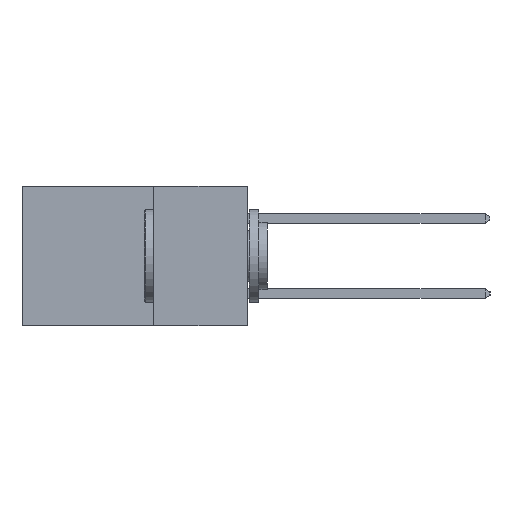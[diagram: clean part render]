
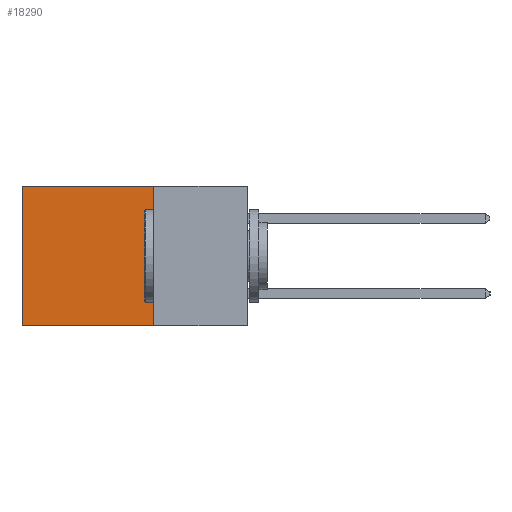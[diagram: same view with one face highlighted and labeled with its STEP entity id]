
A CAD part, left-side view. The second image highlights one B-rep face of the part: STEP entity #18290.
In plain terms, the highlighted planar face has unit normal (-1, 0, 0).
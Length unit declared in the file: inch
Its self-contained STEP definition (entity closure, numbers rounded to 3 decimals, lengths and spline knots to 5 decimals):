
#93 = DIRECTION ( 'NONE',  ( 0., 1., 0. ) ) ;
#675 = CARTESIAN_POINT ( 'NONE',  ( 0.2615, 0.25, -0.37 ) ) ;
#1195 = LINE ( 'NONE', #4726, #13088 ) ;
#2141 = LINE ( 'NONE', #5996, #18094 ) ;
#2378 = VERTEX_POINT ( 'NONE', #8078 ) ;
#2873 = CARTESIAN_POINT ( 'NONE',  ( 0.2615, 0.25, -0.37 ) ) ;
#2901 = DIRECTION ( 'NONE',  ( 0., 0., -1. ) ) ;
#3319 = AXIS2_PLACEMENT_3D ( 'NONE', #675, #13069, #3828 ) ;
#3700 = ORIENTED_EDGE ( 'NONE', *, *, #14038, .F. ) ;
#3828 = DIRECTION ( 'NONE',  ( 0., 0., -1. ) ) ;
#4396 = CARTESIAN_POINT ( 'NONE',  ( 0.2615, 0.25, -0.37 ) ) ;
#4618 = CARTESIAN_POINT ( 'NONE',  ( 0.2615, 0.25, 0. ) ) ;
#4726 = CARTESIAN_POINT ( 'NONE',  ( 0.2615, 0.25, 0. ) ) ;
#4954 = EDGE_CURVE ( 'NONE', #18662, #7941, #1195, .T. ) ;
#5758 = CARTESIAN_POINT ( 'NONE',  ( 0.2615, 0.6, 0. ) ) ;
#5993 = DIRECTION ( 'NONE',  ( 0., 1., 0. ) ) ;
#5996 = CARTESIAN_POINT ( 'NONE',  ( 0.2615, 0.6, -0.37 ) ) ;
#6264 = ORIENTED_EDGE ( 'NONE', *, *, #4954, .T. ) ;
#6842 = PLANE ( 'NONE',  #3319 ) ;
#6877 = EDGE_CURVE ( 'NONE', #7941, #2378, #2141, .T. ) ;
#7016 = LINE ( 'NONE', #2873, #18371 ) ;
#7885 = VERTEX_POINT ( 'NONE', #10334 ) ;
#7941 = VERTEX_POINT ( 'NONE', #5758 ) ;
#8078 = CARTESIAN_POINT ( 'NONE',  ( 0.2615, 0.6, -0.37 ) ) ;
#9812 = LINE ( 'NONE', #4396, #17549 ) ;
#10334 = CARTESIAN_POINT ( 'NONE',  ( 0.2615, 0.25, -0.37 ) ) ;
#10486 = EDGE_CURVE ( 'NONE', #7885, #2378, #7016, .T. ) ;
#11568 = FACE_OUTER_BOUND ( 'NONE', #11969, .T. ) ;
#11969 = EDGE_LOOP ( 'NONE', ( #12447, #16387, #3700, #6264 ) ) ;
#12447 = ORIENTED_EDGE ( 'NONE', *, *, #6877, .T. ) ;
#13069 = DIRECTION ( 'NONE',  ( 1., 0., 0. ) ) ;
#13088 = VECTOR ( 'NONE', #93, 39.37008 ) ;
#14038 = EDGE_CURVE ( 'NONE', #18662, #7885, #9812, .T. ) ;
#16387 = ORIENTED_EDGE ( 'NONE', *, *, #10486, .F. ) ;
#16791 = DIRECTION ( 'NONE',  ( 0., 0., -1. ) ) ;
#17549 = VECTOR ( 'NONE', #2901, 39.37008 ) ;
#18094 = VECTOR ( 'NONE', #16791, 39.37008 ) ;
#18290 = ADVANCED_FACE ( 'NONE', ( #11568 ), #6842, .F. ) ;
#18371 = VECTOR ( 'NONE', #5993, 39.37008 ) ;
#18662 = VERTEX_POINT ( 'NONE', #4618 ) ;
